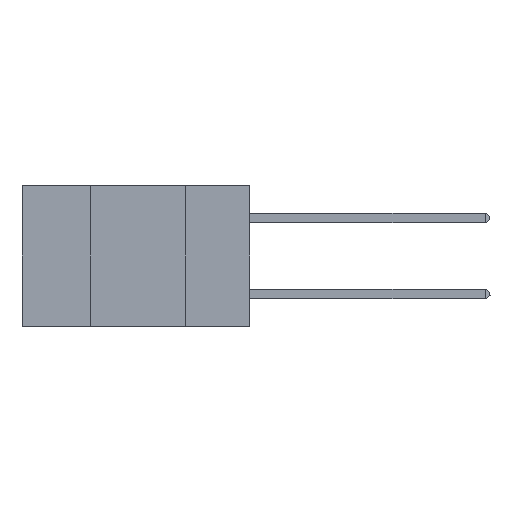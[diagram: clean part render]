
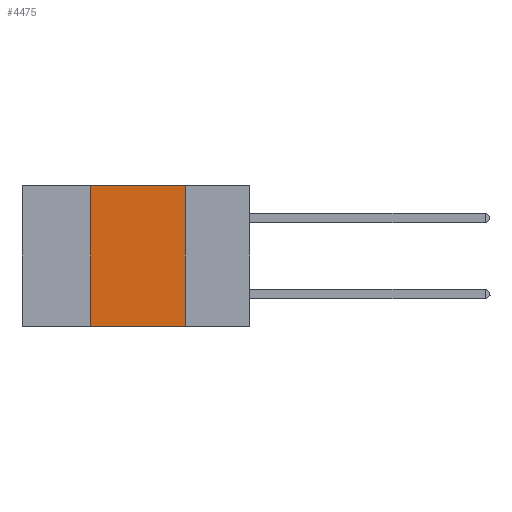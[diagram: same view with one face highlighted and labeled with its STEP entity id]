
A CAD part, left-side view. The second image highlights one B-rep face of the part: STEP entity #4475.
In plain terms, the highlighted planar face has unit normal (-1, 0, 0).
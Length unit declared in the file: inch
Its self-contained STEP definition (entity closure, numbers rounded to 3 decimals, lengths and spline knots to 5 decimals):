
#500 = LINE ( 'NONE', #16152, #6477 ) ;
#539 = CARTESIAN_POINT ( 'NONE',  ( 0., 0.6, 0. ) ) ;
#921 = DIRECTION ( 'NONE',  ( 0., -1., 0. ) ) ;
#3601 = EDGE_CURVE ( 'NONE', #10769, #29218, #8754, .T. ) ;
#4475 = ADVANCED_FACE ( 'NONE', ( #13122 ), #33069, .F. ) ;
#6468 = EDGE_CURVE ( 'NONE', #29218, #12933, #11099, .T. ) ;
#6477 = VECTOR ( 'NONE', #921, 39.37008 ) ;
#7177 = VECTOR ( 'NONE', #18574, 39.37008 ) ;
#8754 = LINE ( 'NONE', #539, #7177 ) ;
#9479 = ORIENTED_EDGE ( 'NONE', *, *, #6468, .F. ) ;
#10007 = DIRECTION ( 'NONE',  ( 0., 0., -1. ) ) ;
#10769 = VERTEX_POINT ( 'NONE', #27161 ) ;
#11099 = LINE ( 'NONE', #26528, #19855 ) ;
#11709 = AXIS2_PLACEMENT_3D ( 'NONE', #20270, #20162, #10007 ) ;
#12639 = ORIENTED_EDGE ( 'NONE', *, *, #22868, .T. ) ;
#12933 = VERTEX_POINT ( 'NONE', #20629 ) ;
#13122 = FACE_OUTER_BOUND ( 'NONE', #31880, .T. ) ;
#15129 = ORIENTED_EDGE ( 'NONE', *, *, #25436, .F. ) ;
#16152 = CARTESIAN_POINT ( 'NONE',  ( 0., 0.6, -0.37 ) ) ;
#16312 = DIRECTION ( 'NONE',  ( 0., 0., -1. ) ) ;
#18574 = DIRECTION ( 'NONE',  ( 0., -1., 0. ) ) ;
#19855 = VECTOR ( 'NONE', #16312, 39.37008 ) ;
#20162 = DIRECTION ( 'NONE',  ( 1., 0., 0. ) ) ;
#20252 = CARTESIAN_POINT ( 'NONE',  ( 0., 0.17, 0. ) ) ;
#20270 = CARTESIAN_POINT ( 'NONE',  ( 0., 0.6, 0. ) ) ;
#20629 = CARTESIAN_POINT ( 'NONE',  ( 0., 0.17, -0.37 ) ) ;
#22868 = EDGE_CURVE ( 'NONE', #26634, #12933, #500, .T. ) ;
#25436 = EDGE_CURVE ( 'NONE', #26634, #10769, #26099, .T. ) ;
#25716 = VECTOR ( 'NONE', #25813, 39.37008 ) ;
#25813 = DIRECTION ( 'NONE',  ( 0., 0., 1. ) ) ;
#26099 = LINE ( 'NONE', #26142, #25716 ) ;
#26142 = CARTESIAN_POINT ( 'NONE',  ( 0., 0.42, 0. ) ) ;
#26528 = CARTESIAN_POINT ( 'NONE',  ( 0., 0.17, 0. ) ) ;
#26634 = VERTEX_POINT ( 'NONE', #30840 ) ;
#27161 = CARTESIAN_POINT ( 'NONE',  ( 0., 0.42, 0. ) ) ;
#29218 = VERTEX_POINT ( 'NONE', #20252 ) ;
#30840 = CARTESIAN_POINT ( 'NONE',  ( 0., 0.42, -0.37 ) ) ;
#31880 = EDGE_LOOP ( 'NONE', ( #9479, #32790, #15129, #12639 ) ) ;
#32790 = ORIENTED_EDGE ( 'NONE', *, *, #3601, .F. ) ;
#33069 = PLANE ( 'NONE',  #11709 ) ;
